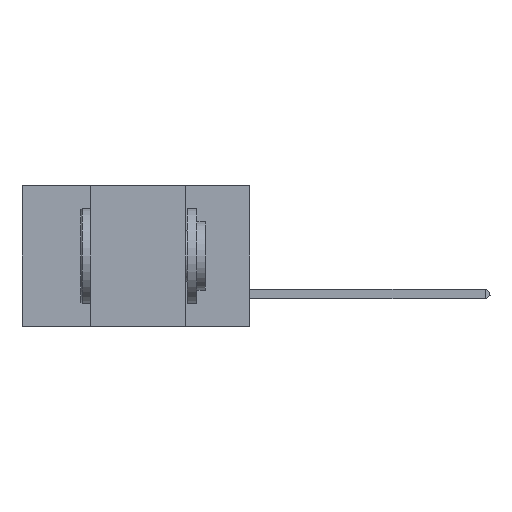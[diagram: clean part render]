
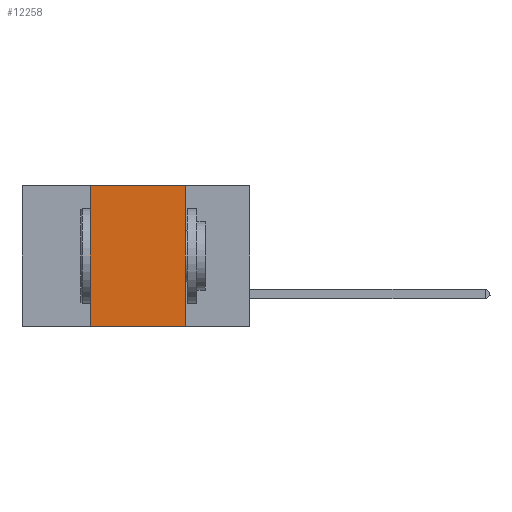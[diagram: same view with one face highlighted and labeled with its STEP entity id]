
A CAD part, left-side view. The second image highlights one B-rep face of the part: STEP entity #12258.
In plain terms, the highlighted planar face has unit normal (-1, 0, 0).
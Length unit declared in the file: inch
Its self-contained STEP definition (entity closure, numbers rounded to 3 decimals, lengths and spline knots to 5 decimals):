
#437 = DIRECTION ( 'NONE',  ( 0., -1., 0. ) ) ;
#621 = EDGE_CURVE ( 'NONE', #9640, #12574, #10750, .T. ) ;
#675 = CARTESIAN_POINT ( 'NONE',  ( 0., 0.42, 0. ) ) ;
#1319 = CARTESIAN_POINT ( 'NONE',  ( 0., 0.42, -0.37 ) ) ;
#1830 = VERTEX_POINT ( 'NONE', #1319 ) ;
#2578 = ORIENTED_EDGE ( 'NONE', *, *, #6661, .F. ) ;
#2757 = FACE_OUTER_BOUND ( 'NONE', #14656, .T. ) ;
#3397 = CARTESIAN_POINT ( 'NONE',  ( 0., 0.6, 0. ) ) ;
#3645 = AXIS2_PLACEMENT_3D ( 'NONE', #15638, #10193, #11639 ) ;
#3842 = CARTESIAN_POINT ( 'NONE',  ( 0., 0.17, 0. ) ) ;
#4058 = CARTESIAN_POINT ( 'NONE',  ( 0., 0.17, 0. ) ) ;
#5333 = LINE ( 'NONE', #12420, #9305 ) ;
#5437 = ORIENTED_EDGE ( 'NONE', *, *, #16033, .F. ) ;
#6661 = EDGE_CURVE ( 'NONE', #7648, #9640, #11695, .T. ) ;
#7648 = VERTEX_POINT ( 'NONE', #675 ) ;
#8144 = CARTESIAN_POINT ( 'NONE',  ( 0., 0.42, 0. ) ) ;
#9305 = VECTOR ( 'NONE', #13643, 39.37008 ) ;
#9640 = VERTEX_POINT ( 'NONE', #3842 ) ;
#10109 = ORIENTED_EDGE ( 'NONE', *, *, #11146, .T. ) ;
#10144 = VECTOR ( 'NONE', #11253, 39.37008 ) ;
#10193 = DIRECTION ( 'NONE',  ( 1., 0., 0. ) ) ;
#10750 = LINE ( 'NONE', #4058, #11649 ) ;
#11146 = EDGE_CURVE ( 'NONE', #1830, #12574, #5333, .T. ) ;
#11175 = CARTESIAN_POINT ( 'NONE',  ( 0., 0.17, -0.37 ) ) ;
#11253 = DIRECTION ( 'NONE',  ( 0., 0., 1. ) ) ;
#11512 = PLANE ( 'NONE',  #3645 ) ;
#11639 = DIRECTION ( 'NONE',  ( 0., 0., -1. ) ) ;
#11649 = VECTOR ( 'NONE', #12619, 39.37008 ) ;
#11695 = LINE ( 'NONE', #3397, #14519 ) ;
#12258 = ADVANCED_FACE ( 'NONE', ( #2757 ), #11512, .F. ) ;
#12420 = CARTESIAN_POINT ( 'NONE',  ( 0., 0.6, -0.37 ) ) ;
#12574 = VERTEX_POINT ( 'NONE', #11175 ) ;
#12619 = DIRECTION ( 'NONE',  ( 0., 0., -1. ) ) ;
#13643 = DIRECTION ( 'NONE',  ( 0., -1., 0. ) ) ;
#14519 = VECTOR ( 'NONE', #437, 39.37008 ) ;
#14656 = EDGE_LOOP ( 'NONE', ( #17926, #2578, #5437, #10109 ) ) ;
#15638 = CARTESIAN_POINT ( 'NONE',  ( 0., 0.6, 0. ) ) ;
#16033 = EDGE_CURVE ( 'NONE', #1830, #7648, #17586, .T. ) ;
#17586 = LINE ( 'NONE', #8144, #10144 ) ;
#17926 = ORIENTED_EDGE ( 'NONE', *, *, #621, .F. ) ;
